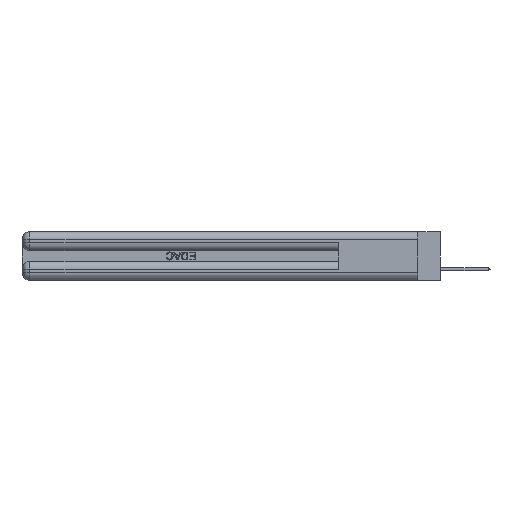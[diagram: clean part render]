
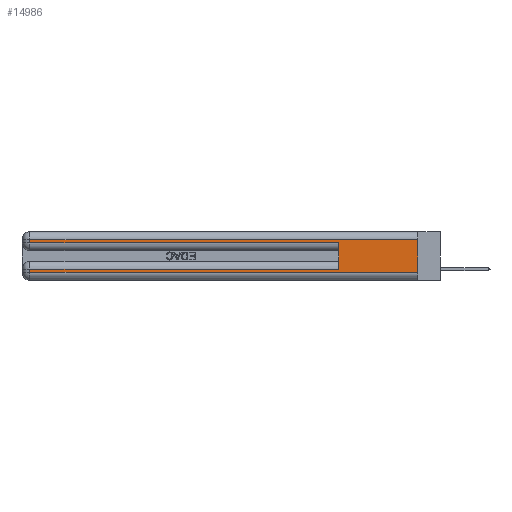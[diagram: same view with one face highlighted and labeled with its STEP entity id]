
A CAD part, left-side view. The second image highlights one B-rep face of the part: STEP entity #14986.
In plain terms, the highlighted planar face has unit normal (-1, 0, 0).
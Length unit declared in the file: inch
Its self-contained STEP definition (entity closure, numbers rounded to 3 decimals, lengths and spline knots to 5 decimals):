
#1087 = EDGE_CURVE ( 'NONE', #25760, #23231, #34023, .T. ) ;
#1475 = AXIS2_PLACEMENT_3D ( 'NONE', #5139, #42977, #5777 ) ;
#4121 = EDGE_CURVE ( 'NONE', #11376, #42490, #40657, .T. ) ;
#4253 = CARTESIAN_POINT ( 'NONE',  ( 0., 2.94, 0.285 ) ) ;
#4388 = VECTOR ( 'NONE', #9301, 39.37008 ) ;
#4542 = CARTESIAN_POINT ( 'NONE',  ( 0., 2.94, 0.06 ) ) ;
#4582 = EDGE_CURVE ( 'NONE', #22442, #11376, #12127, .T. ) ;
#4773 = LINE ( 'NONE', #12439, #6494 ) ;
#4834 = DIRECTION ( 'NONE',  ( 0., -1., 0. ) ) ;
#5139 = CARTESIAN_POINT ( 'NONE',  ( 0., 0., 0.37 ) ) ;
#5220 = DIRECTION ( 'NONE',  ( 0., 1., 0. ) ) ;
#5777 = DIRECTION ( 'NONE',  ( 0., 0., -1. ) ) ;
#6494 = VECTOR ( 'NONE', #38456, 39.37008 ) ;
#9301 = DIRECTION ( 'NONE',  ( 0., 1., 0. ) ) ;
#9794 = VECTOR ( 'NONE', #5220, 39.37008 ) ;
#11008 = VECTOR ( 'NONE', #41154, 39.37008 ) ;
#11376 = VERTEX_POINT ( 'NONE', #24953 ) ;
#11930 = VECTOR ( 'NONE', #28310, 39.37008 ) ;
#12127 = LINE ( 'NONE', #23886, #9794 ) ;
#12439 = CARTESIAN_POINT ( 'NONE',  ( 0., 0., 0.285 ) ) ;
#12614 = CARTESIAN_POINT ( 'NONE',  ( 0., 2.94, 0.37 ) ) ;
#13112 = LINE ( 'NONE', #31562, #11930 ) ;
#13141 = LINE ( 'NONE', #12614, #16055 ) ;
#13420 = EDGE_CURVE ( 'NONE', #15263, #43442, #22727, .T. ) ;
#13798 = ORIENTED_EDGE ( 'NONE', *, *, #36654, .T. ) ;
#14986 = ADVANCED_FACE ( 'NONE', ( #22497 ), #46492, .F. ) ;
#15263 = VERTEX_POINT ( 'NONE', #4542 ) ;
#16055 = VECTOR ( 'NONE', #31268, 39.37008 ) ;
#16411 = EDGE_CURVE ( 'NONE', #25760, #38792, #13112, .T. ) ;
#17469 = CARTESIAN_POINT ( 'NONE',  ( 0., 0., 0.085 ) ) ;
#17823 = EDGE_LOOP ( 'NONE', ( #44780, #26721, #35746, #13798, #18405, #28024, #43407, #25488 ) ) ;
#18405 = ORIENTED_EDGE ( 'NONE', *, *, #16411, .F. ) ;
#22134 = CARTESIAN_POINT ( 'NONE',  ( 0., 2.94, 0.37 ) ) ;
#22442 = VERTEX_POINT ( 'NONE', #40016 ) ;
#22497 = FACE_OUTER_BOUND ( 'NONE', #17823, .T. ) ;
#22727 = LINE ( 'NONE', #23338, #46507 ) ;
#23231 = VERTEX_POINT ( 'NONE', #41178 ) ;
#23338 = CARTESIAN_POINT ( 'NONE',  ( 0., 0., 0.06 ) ) ;
#23886 = CARTESIAN_POINT ( 'NONE',  ( 0., 0., 0.31 ) ) ;
#24788 = DIRECTION ( 'NONE',  ( 0., 0., -1. ) ) ;
#24953 = CARTESIAN_POINT ( 'NONE',  ( 0., 2.94, 0.31 ) ) ;
#25488 = ORIENTED_EDGE ( 'NONE', *, *, #13420, .T. ) ;
#25760 = VERTEX_POINT ( 'NONE', #33879 ) ;
#26721 = ORIENTED_EDGE ( 'NONE', *, *, #4582, .T. ) ;
#27595 = EDGE_CURVE ( 'NONE', #23231, #15263, #13141, .T. ) ;
#28024 = ORIENTED_EDGE ( 'NONE', *, *, #1087, .T. ) ;
#28111 = CARTESIAN_POINT ( 'NONE',  ( 0., 0.6, 0.285 ) ) ;
#28191 = CARTESIAN_POINT ( 'NONE',  ( 0., 0., 0.06 ) ) ;
#28310 = DIRECTION ( 'NONE',  ( 0., 0., 1. ) ) ;
#31268 = DIRECTION ( 'NONE',  ( 0., 0., -1. ) ) ;
#31562 = CARTESIAN_POINT ( 'NONE',  ( 0., 0.6, 0.145 ) ) ;
#33879 = CARTESIAN_POINT ( 'NONE',  ( 0., 0.6, 0.085 ) ) ;
#34023 = LINE ( 'NONE', #17469, #4388 ) ;
#35479 = VECTOR ( 'NONE', #24788, 39.37008 ) ;
#35746 = ORIENTED_EDGE ( 'NONE', *, *, #4121, .T. ) ;
#36654 = EDGE_CURVE ( 'NONE', #42490, #38792, #4773, .T. ) ;
#38456 = DIRECTION ( 'NONE',  ( 0., -1., 0. ) ) ;
#38792 = VERTEX_POINT ( 'NONE', #28111 ) ;
#40016 = CARTESIAN_POINT ( 'NONE',  ( 0., 0., 0.31 ) ) ;
#40657 = LINE ( 'NONE', #22134, #11008 ) ;
#41154 = DIRECTION ( 'NONE',  ( 0., 0., -1. ) ) ;
#41178 = CARTESIAN_POINT ( 'NONE',  ( 0., 2.94, 0.085 ) ) ;
#42490 = VERTEX_POINT ( 'NONE', #4253 ) ;
#42977 = DIRECTION ( 'NONE',  ( 1., 0., 0. ) ) ;
#43407 = ORIENTED_EDGE ( 'NONE', *, *, #27595, .T. ) ;
#43442 = VERTEX_POINT ( 'NONE', #28191 ) ;
#43474 = EDGE_CURVE ( 'NONE', #22442, #43442, #47605, .T. ) ;
#44780 = ORIENTED_EDGE ( 'NONE', *, *, #43474, .F. ) ;
#46492 = PLANE ( 'NONE',  #1475 ) ;
#46507 = VECTOR ( 'NONE', #4834, 39.37008 ) ;
#46987 = CARTESIAN_POINT ( 'NONE',  ( 0., 0., 0.37 ) ) ;
#47605 = LINE ( 'NONE', #46987, #35479 ) ;
